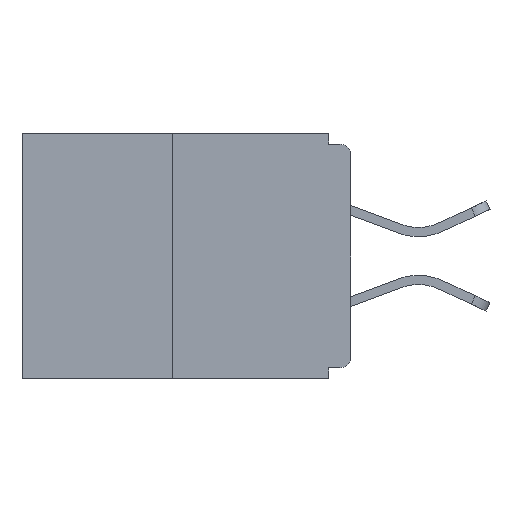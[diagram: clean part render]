
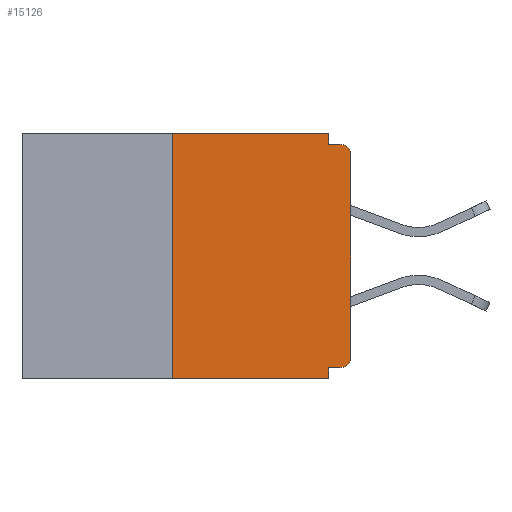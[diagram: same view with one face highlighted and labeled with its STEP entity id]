
A CAD part, left-side view. The second image highlights one B-rep face of the part: STEP entity #15126.
In plain terms, the highlighted planar face has unit normal (-1, 0, 0).
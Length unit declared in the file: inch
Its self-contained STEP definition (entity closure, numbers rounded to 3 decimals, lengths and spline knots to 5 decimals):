
#27 = EDGE_CURVE ( 'NONE', #2605, #8615, #14040, .T. ) ;
#218 = VECTOR ( 'NONE', #12538, 39.37008 ) ;
#260 = CARTESIAN_POINT ( 'NONE',  ( 0., 0., -0.328 ) ) ;
#578 = VECTOR ( 'NONE', #11254, 39.37008 ) ;
#707 = VERTEX_POINT ( 'NONE', #1378 ) ;
#1166 = LINE ( 'NONE', #10424, #578 ) ;
#1264 = CARTESIAN_POINT ( 'NONE',  ( 0., 0., -0.313 ) ) ;
#1277 = VERTEX_POINT ( 'NONE', #9299 ) ;
#1378 = CARTESIAN_POINT ( 'NONE',  ( 0., 0.25, -0.343 ) ) ;
#1396 = CARTESIAN_POINT ( 'NONE',  ( 0., 0.031, 0. ) ) ;
#1458 = DIRECTION ( 'NONE',  ( 0., 1., 0. ) ) ;
#1809 = CARTESIAN_POINT ( 'NONE',  ( 0., 0.46, 0. ) ) ;
#1850 = DIRECTION ( 'NONE',  ( -1., 0., 0. ) ) ;
#1942 = CARTESIAN_POINT ( 'NONE',  ( 0., 0.015, -0.313 ) ) ;
#2103 = FACE_OUTER_BOUND ( 'NONE', #13670, .T. ) ;
#2237 = EDGE_CURVE ( 'NONE', #3391, #1277, #5871, .T. ) ;
#2486 = CARTESIAN_POINT ( 'NONE',  ( 0., 0.031, -0.343 ) ) ;
#2605 = VERTEX_POINT ( 'NONE', #1396 ) ;
#2641 = AXIS2_PLACEMENT_3D ( 'NONE', #1942, #1850, #11200 ) ;
#2657 = CARTESIAN_POINT ( 'NONE',  ( 0., 0.031, -0.015 ) ) ;
#2914 = CARTESIAN_POINT ( 'NONE',  ( 0., 0.031, -0.328 ) ) ;
#2989 = ORIENTED_EDGE ( 'NONE', *, *, #11255, .T. ) ;
#3131 = AXIS2_PLACEMENT_3D ( 'NONE', #12784, #12947, #6280 ) ;
#3391 = VERTEX_POINT ( 'NONE', #1264 ) ;
#3515 = CARTESIAN_POINT ( 'NONE',  ( 0., 0., 0. ) ) ;
#3780 = VERTEX_POINT ( 'NONE', #8988 ) ;
#3956 = EDGE_CURVE ( 'NONE', #16429, #16548, #9851, .T. ) ;
#4141 = EDGE_CURVE ( 'NONE', #8615, #3780, #1166, .T. ) ;
#4883 = PLANE ( 'NONE',  #3131 ) ;
#5444 = CARTESIAN_POINT ( 'NONE',  ( 0., 0.015, -0.328 ) ) ;
#5636 = ORIENTED_EDGE ( 'NONE', *, *, #6824, .F. ) ;
#5735 = LINE ( 'NONE', #1809, #7074 ) ;
#5871 = LINE ( 'NONE', #3515, #218 ) ;
#6165 = EDGE_CURVE ( 'NONE', #13207, #2605, #5735, .T. ) ;
#6280 = DIRECTION ( 'NONE',  ( 0., 0., -1. ) ) ;
#6726 = LINE ( 'NONE', #11733, #10475 ) ;
#6824 = EDGE_CURVE ( 'NONE', #16548, #16363, #10178, .T. ) ;
#7074 = VECTOR ( 'NONE', #15038, 39.37008 ) ;
#7384 = CARTESIAN_POINT ( 'NONE',  ( 0., 0.031, 0. ) ) ;
#7423 = ORIENTED_EDGE ( 'NONE', *, *, #9119, .T. ) ;
#7486 = CARTESIAN_POINT ( 'NONE',  ( 0., 0.031, -0.343 ) ) ;
#7645 = EDGE_CURVE ( 'NONE', #707, #16363, #6726, .T. ) ;
#7655 = CARTESIAN_POINT ( 'NONE',  ( 0., 0.25, 0. ) ) ;
#8142 = VECTOR ( 'NONE', #12724, 39.37008 ) ;
#8615 = VERTEX_POINT ( 'NONE', #2657 ) ;
#8759 = VECTOR ( 'NONE', #11497, 39.37008 ) ;
#8988 = CARTESIAN_POINT ( 'NONE',  ( 0., 0.015, -0.015 ) ) ;
#9119 = EDGE_CURVE ( 'NONE', #16429, #3391, #16384, .T. ) ;
#9299 = CARTESIAN_POINT ( 'NONE',  ( 0., 0., -0.03 ) ) ;
#9851 = LINE ( 'NONE', #260, #12699 ) ;
#10178 = LINE ( 'NONE', #7486, #8759 ) ;
#10334 = ORIENTED_EDGE ( 'NONE', *, *, #3956, .F. ) ;
#10421 = DIRECTION ( 'NONE',  ( 0., 0., 1. ) ) ;
#10424 = CARTESIAN_POINT ( 'NONE',  ( 0., 0., -0.015 ) ) ;
#10475 = VECTOR ( 'NONE', #10657, 39.37008 ) ;
#10623 = ORIENTED_EDGE ( 'NONE', *, *, #16812, .F. ) ;
#10657 = DIRECTION ( 'NONE',  ( 0., -1., 0. ) ) ;
#10980 = DIRECTION ( 'NONE',  ( 0., 0., -1. ) ) ;
#11200 = DIRECTION ( 'NONE',  ( 0., 0., -1. ) ) ;
#11238 = ORIENTED_EDGE ( 'NONE', *, *, #6165, .F. ) ;
#11254 = DIRECTION ( 'NONE',  ( 0., -1., 0. ) ) ;
#11255 = EDGE_CURVE ( 'NONE', #1277, #3780, #12801, .T. ) ;
#11497 = DIRECTION ( 'NONE',  ( 0., 0., -1. ) ) ;
#11733 = CARTESIAN_POINT ( 'NONE',  ( 0., 0.46, -0.343 ) ) ;
#12538 = DIRECTION ( 'NONE',  ( 0., 0., 1. ) ) ;
#12699 = VECTOR ( 'NONE', #1458, 39.37008 ) ;
#12724 = DIRECTION ( 'NONE',  ( 0., 0., -1. ) ) ;
#12784 = CARTESIAN_POINT ( 'NONE',  ( 0., 0.46, 0. ) ) ;
#12801 = CIRCLE ( 'NONE', #15022, 0.015 ) ;
#12947 = DIRECTION ( 'NONE',  ( 1., 0., 0. ) ) ;
#13207 = VERTEX_POINT ( 'NONE', #15911 ) ;
#13233 = ORIENTED_EDGE ( 'NONE', *, *, #7645, .T. ) ;
#13670 = EDGE_LOOP ( 'NONE', ( #11238, #10623, #13233, #5636, #10334, #7423, #14279, #2989, #16977, #14059 ) ) ;
#14040 = LINE ( 'NONE', #7384, #8142 ) ;
#14059 = ORIENTED_EDGE ( 'NONE', *, *, #27, .F. ) ;
#14279 = ORIENTED_EDGE ( 'NONE', *, *, #2237, .T. ) ;
#14838 = CARTESIAN_POINT ( 'NONE',  ( 0., 0.015, -0.03 ) ) ;
#15022 = AXIS2_PLACEMENT_3D ( 'NONE', #14838, #16161, #10980 ) ;
#15038 = DIRECTION ( 'NONE',  ( 0., -1., 0. ) ) ;
#15126 = ADVANCED_FACE ( 'NONE', ( #2103 ), #4883, .F. ) ;
#15699 = LINE ( 'NONE', #7655, #16596 ) ;
#15911 = CARTESIAN_POINT ( 'NONE',  ( 0., 0.25, 0. ) ) ;
#16161 = DIRECTION ( 'NONE',  ( -1., 0., 0. ) ) ;
#16363 = VERTEX_POINT ( 'NONE', #2486 ) ;
#16384 = CIRCLE ( 'NONE', #2641, 0.015 ) ;
#16429 = VERTEX_POINT ( 'NONE', #5444 ) ;
#16548 = VERTEX_POINT ( 'NONE', #2914 ) ;
#16596 = VECTOR ( 'NONE', #10421, 39.37008 ) ;
#16812 = EDGE_CURVE ( 'NONE', #707, #13207, #15699, .T. ) ;
#16977 = ORIENTED_EDGE ( 'NONE', *, *, #4141, .F. ) ;
